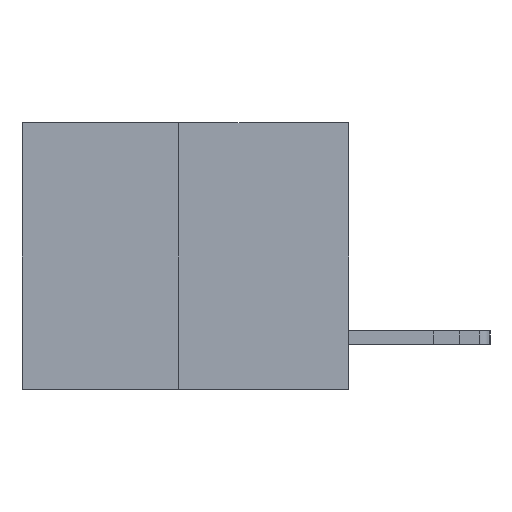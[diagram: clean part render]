
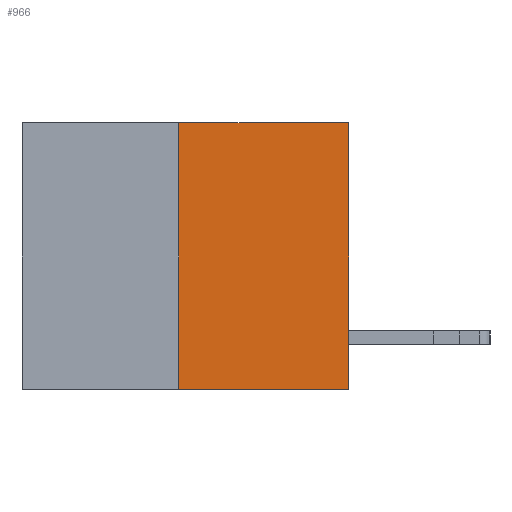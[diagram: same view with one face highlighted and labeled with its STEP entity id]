
A CAD part, left-side view. The second image highlights one B-rep face of the part: STEP entity #966.
In plain terms, the highlighted planar face has unit normal (-1, 0, 0).
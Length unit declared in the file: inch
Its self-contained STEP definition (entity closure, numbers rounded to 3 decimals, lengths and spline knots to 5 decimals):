
#436 = VECTOR ( 'NONE', #7288, 39.37008 ) ;
#459 = DIRECTION ( 'NONE',  ( 0., -1., 0. ) ) ;
#703 = VECTOR ( 'NONE', #10448, 39.37008 ) ;
#966 = ADVANCED_FACE ( 'NONE', ( #9277 ), #17726, .F. ) ;
#1317 = LINE ( 'NONE', #9467, #12876 ) ;
#1323 = VERTEX_POINT ( 'NONE', #11165 ) ;
#1386 = ORIENTED_EDGE ( 'NONE', *, *, #3668, .T. ) ;
#2624 = CARTESIAN_POINT ( 'NONE',  ( 0., 0.312, -0.49 ) ) ;
#3140 = VECTOR ( 'NONE', #18607, 39.37008 ) ;
#3597 = LINE ( 'NONE', #17106, #3140 ) ;
#3668 = EDGE_CURVE ( 'NONE', #14510, #1323, #3597, .T. ) ;
#4350 = ORIENTED_EDGE ( 'NONE', *, *, #9730, .F. ) ;
#4758 = LINE ( 'NONE', #17976, #703 ) ;
#5843 = VERTEX_POINT ( 'NONE', #16479 ) ;
#6882 = AXIS2_PLACEMENT_3D ( 'NONE', #16097, #13107, #14427 ) ;
#7288 = DIRECTION ( 'NONE',  ( 0., -1., 0. ) ) ;
#7953 = EDGE_CURVE ( 'NONE', #5843, #1323, #1317, .T. ) ;
#9103 = EDGE_LOOP ( 'NONE', ( #4350, #13515, #1386, #12469 ) ) ;
#9277 = FACE_OUTER_BOUND ( 'NONE', #9103, .T. ) ;
#9467 = CARTESIAN_POINT ( 'NONE',  ( 0., 0.6, 0. ) ) ;
#9730 = EDGE_CURVE ( 'NONE', #14477, #5843, #4758, .T. ) ;
#9964 = EDGE_CURVE ( 'NONE', #14477, #14510, #16744, .T. ) ;
#10448 = DIRECTION ( 'NONE',  ( 0., 0., 1. ) ) ;
#11165 = CARTESIAN_POINT ( 'NONE',  ( 0., 0., 0. ) ) ;
#12469 = ORIENTED_EDGE ( 'NONE', *, *, #7953, .F. ) ;
#12876 = VECTOR ( 'NONE', #459, 39.37008 ) ;
#13107 = DIRECTION ( 'NONE',  ( 1., 0., 0. ) ) ;
#13515 = ORIENTED_EDGE ( 'NONE', *, *, #9964, .T. ) ;
#14427 = DIRECTION ( 'NONE',  ( 0., 0., -1. ) ) ;
#14477 = VERTEX_POINT ( 'NONE', #2624 ) ;
#14510 = VERTEX_POINT ( 'NONE', #18089 ) ;
#16097 = CARTESIAN_POINT ( 'NONE',  ( 0., 0.6, 0. ) ) ;
#16459 = CARTESIAN_POINT ( 'NONE',  ( 0., 0.6, -0.49 ) ) ;
#16479 = CARTESIAN_POINT ( 'NONE',  ( 0., 0.312, 0. ) ) ;
#16744 = LINE ( 'NONE', #16459, #436 ) ;
#17106 = CARTESIAN_POINT ( 'NONE',  ( 0., 0., 0. ) ) ;
#17726 = PLANE ( 'NONE',  #6882 ) ;
#17976 = CARTESIAN_POINT ( 'NONE',  ( 0., 0.312, -0.49 ) ) ;
#18089 = CARTESIAN_POINT ( 'NONE',  ( 0., 0., -0.49 ) ) ;
#18607 = DIRECTION ( 'NONE',  ( 0., 0., 1. ) ) ;
